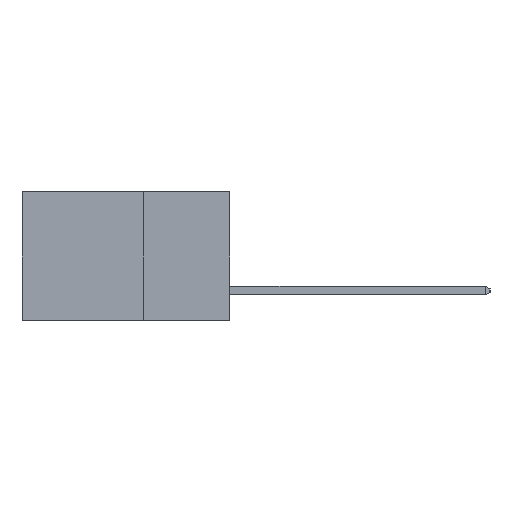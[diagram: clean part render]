
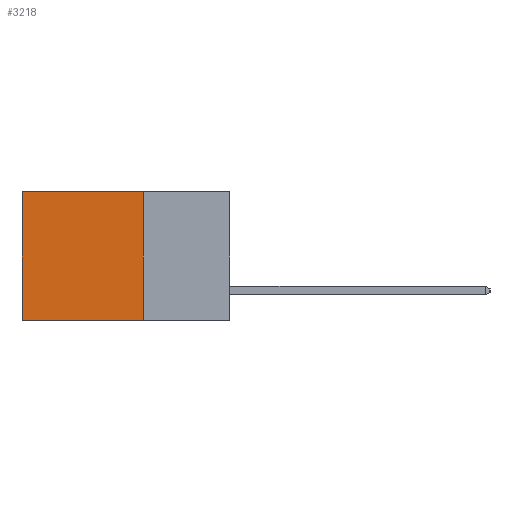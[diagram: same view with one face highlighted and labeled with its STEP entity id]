
A CAD part, left-side view. The second image highlights one B-rep face of the part: STEP entity #3218.
In plain terms, the highlighted planar face has unit normal (-1, 0, 0).
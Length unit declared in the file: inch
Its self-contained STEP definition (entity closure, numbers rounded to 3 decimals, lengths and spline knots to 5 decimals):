
#26 = VECTOR ( 'NONE', #8182, 39.37008 ) ;
#154 = EDGE_LOOP ( 'NONE', ( #6196, #20590, #13769, #2765 ) ) ;
#706 = LINE ( 'NONE', #8354, #26 ) ;
#1644 = VERTEX_POINT ( 'NONE', #14327 ) ;
#2765 = ORIENTED_EDGE ( 'NONE', *, *, #3208, .T. ) ;
#2801 = CARTESIAN_POINT ( 'NONE',  ( 0.2615, 0.25, -0.37 ) ) ;
#2806 = FACE_OUTER_BOUND ( 'NONE', #154, .T. ) ;
#3208 = EDGE_CURVE ( 'NONE', #15226, #4780, #22183, .T. ) ;
#3218 = ADVANCED_FACE ( 'NONE', ( #2806 ), #23650, .F. ) ;
#4662 = VECTOR ( 'NONE', #17350, 39.37008 ) ;
#4780 = VERTEX_POINT ( 'NONE', #5460 ) ;
#5460 = CARTESIAN_POINT ( 'NONE',  ( 0.2615, 0.6, 0. ) ) ;
#6196 = ORIENTED_EDGE ( 'NONE', *, *, #7928, .T. ) ;
#6560 = AXIS2_PLACEMENT_3D ( 'NONE', #23675, #23592, #23587 ) ;
#7928 = EDGE_CURVE ( 'NONE', #4780, #1644, #9954, .T. ) ;
#8182 = DIRECTION ( 'NONE',  ( 0., 0., -1. ) ) ;
#8354 = CARTESIAN_POINT ( 'NONE',  ( 0.2615, 0.25, -0.37 ) ) ;
#8439 = EDGE_CURVE ( 'NONE', #15474, #1644, #23942, .T. ) ;
#8508 = EDGE_CURVE ( 'NONE', #15226, #15474, #706, .T. ) ;
#9954 = LINE ( 'NONE', #17400, #4662 ) ;
#9963 = CARTESIAN_POINT ( 'NONE',  ( 0.2615, 0.25, -0.37 ) ) ;
#10015 = DIRECTION ( 'NONE',  ( 0., 1., 0. ) ) ;
#13769 = ORIENTED_EDGE ( 'NONE', *, *, #8508, .F. ) ;
#14327 = CARTESIAN_POINT ( 'NONE',  ( 0.2615, 0.6, -0.37 ) ) ;
#15226 = VERTEX_POINT ( 'NONE', #16143 ) ;
#15474 = VERTEX_POINT ( 'NONE', #2801 ) ;
#16143 = CARTESIAN_POINT ( 'NONE',  ( 0.2615, 0.25, 0. ) ) ;
#17009 = VECTOR ( 'NONE', #23727, 39.37008 ) ;
#17350 = DIRECTION ( 'NONE',  ( 0., 0., -1. ) ) ;
#17400 = CARTESIAN_POINT ( 'NONE',  ( 0.2615, 0.6, -0.37 ) ) ;
#19356 = VECTOR ( 'NONE', #10015, 39.37008 ) ;
#20590 = ORIENTED_EDGE ( 'NONE', *, *, #8439, .F. ) ;
#22183 = LINE ( 'NONE', #23753, #17009 ) ;
#23587 = DIRECTION ( 'NONE',  ( 0., 0., -1. ) ) ;
#23592 = DIRECTION ( 'NONE',  ( 1., 0., 0. ) ) ;
#23650 = PLANE ( 'NONE',  #6560 ) ;
#23675 = CARTESIAN_POINT ( 'NONE',  ( 0.2615, 0.25, -0.37 ) ) ;
#23727 = DIRECTION ( 'NONE',  ( 0., 1., 0. ) ) ;
#23753 = CARTESIAN_POINT ( 'NONE',  ( 0.2615, 0.25, 0. ) ) ;
#23942 = LINE ( 'NONE', #9963, #19356 ) ;
